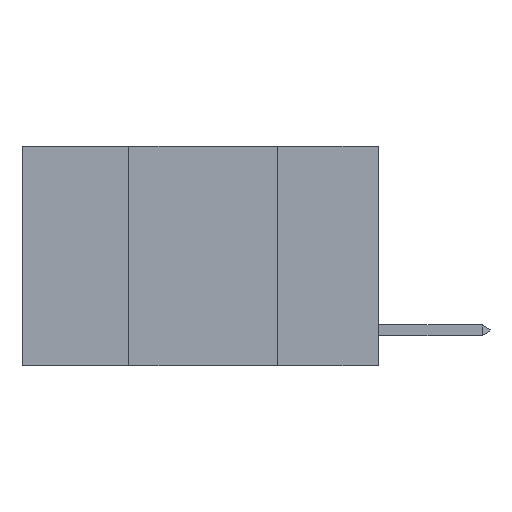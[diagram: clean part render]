
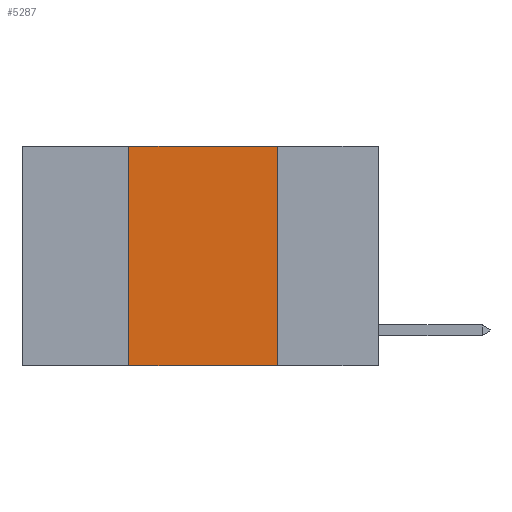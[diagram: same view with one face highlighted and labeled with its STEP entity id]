
A CAD part, left-side view. The second image highlights one B-rep face of the part: STEP entity #5287.
In plain terms, the highlighted planar face has unit normal (-1, 0, 0).
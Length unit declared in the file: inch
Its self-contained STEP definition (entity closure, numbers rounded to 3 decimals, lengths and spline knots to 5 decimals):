
#429 = EDGE_CURVE ( 'NONE', #17213, #1419, #11034, .T. ) ;
#1021 = CARTESIAN_POINT ( 'NONE',  ( 0., 0.17, 0. ) ) ;
#1419 = VERTEX_POINT ( 'NONE', #4182 ) ;
#2092 = AXIS2_PLACEMENT_3D ( 'NONE', #9297, #12265, #9390 ) ;
#2162 = FACE_OUTER_BOUND ( 'NONE', #17933, .T. ) ;
#2347 = PLANE ( 'NONE',  #2092 ) ;
#2359 = LINE ( 'NONE', #3766, #4102 ) ;
#2713 = CARTESIAN_POINT ( 'NONE',  ( 0., 0.42, 0. ) ) ;
#3525 = DIRECTION ( 'NONE',  ( 0., -1., 0. ) ) ;
#3592 = VERTEX_POINT ( 'NONE', #11430 ) ;
#3766 = CARTESIAN_POINT ( 'NONE',  ( 0., 0.42, 0. ) ) ;
#3828 = EDGE_CURVE ( 'NONE', #3592, #1419, #7508, .T. ) ;
#3900 = CARTESIAN_POINT ( 'NONE',  ( 0., 0.6, 0. ) ) ;
#4102 = VECTOR ( 'NONE', #7984, 39.37008 ) ;
#4182 = CARTESIAN_POINT ( 'NONE',  ( 0., 0.17, -0.37 ) ) ;
#4779 = CARTESIAN_POINT ( 'NONE',  ( 0., 0.6, -0.37 ) ) ;
#5250 = ORIENTED_EDGE ( 'NONE', *, *, #429, .F. ) ;
#5287 = ADVANCED_FACE ( 'NONE', ( #2162 ), #2347, .F. ) ;
#6006 = DIRECTION ( 'NONE',  ( 0., -1., 0. ) ) ;
#6496 = VERTEX_POINT ( 'NONE', #2713 ) ;
#6628 = LINE ( 'NONE', #3900, #7363 ) ;
#7363 = VECTOR ( 'NONE', #3525, 39.37008 ) ;
#7508 = LINE ( 'NONE', #4779, #11812 ) ;
#7604 = EDGE_CURVE ( 'NONE', #3592, #6496, #2359, .T. ) ;
#7984 = DIRECTION ( 'NONE',  ( 0., 0., 1. ) ) ;
#9297 = CARTESIAN_POINT ( 'NONE',  ( 0., 0.6, 0. ) ) ;
#9390 = DIRECTION ( 'NONE',  ( 0., 0., -1. ) ) ;
#10398 = ORIENTED_EDGE ( 'NONE', *, *, #3828, .T. ) ;
#11034 = LINE ( 'NONE', #1021, #14269 ) ;
#11162 = ORIENTED_EDGE ( 'NONE', *, *, #7604, .F. ) ;
#11430 = CARTESIAN_POINT ( 'NONE',  ( 0., 0.42, -0.37 ) ) ;
#11812 = VECTOR ( 'NONE', #6006, 39.37008 ) ;
#12265 = DIRECTION ( 'NONE',  ( 1., 0., 0. ) ) ;
#12417 = CARTESIAN_POINT ( 'NONE',  ( 0., 0.17, 0. ) ) ;
#14269 = VECTOR ( 'NONE', #18244, 39.37008 ) ;
#17213 = VERTEX_POINT ( 'NONE', #12417 ) ;
#17907 = ORIENTED_EDGE ( 'NONE', *, *, #17941, .F. ) ;
#17933 = EDGE_LOOP ( 'NONE', ( #5250, #17907, #11162, #10398 ) ) ;
#17941 = EDGE_CURVE ( 'NONE', #6496, #17213, #6628, .T. ) ;
#18244 = DIRECTION ( 'NONE',  ( 0., 0., -1. ) ) ;
